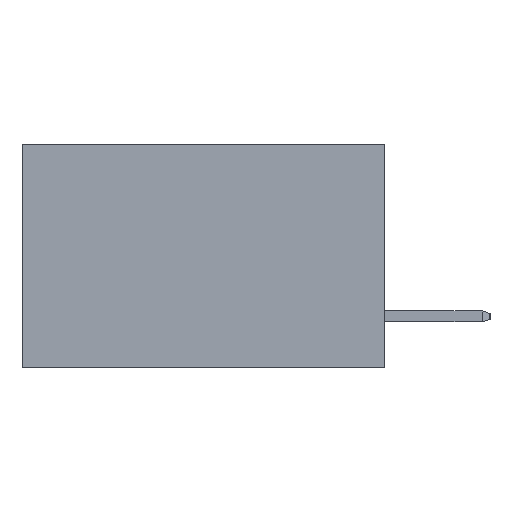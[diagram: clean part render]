
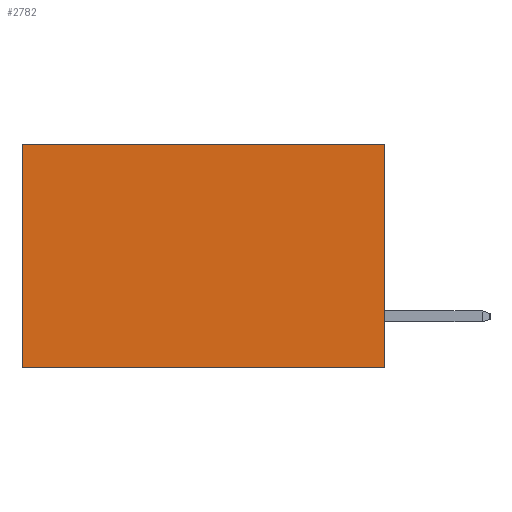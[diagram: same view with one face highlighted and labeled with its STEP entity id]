
A CAD part, left-side view. The second image highlights one B-rep face of the part: STEP entity #2782.
In plain terms, the highlighted planar face has unit normal (-1, 0, 0).
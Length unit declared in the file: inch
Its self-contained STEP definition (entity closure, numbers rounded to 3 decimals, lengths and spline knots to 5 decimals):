
#488 = VECTOR ( 'NONE', #8512, 39.37008 ) ;
#619 = VECTOR ( 'NONE', #1929, 39.37008 ) ;
#1656 = EDGE_CURVE ( 'NONE', #5287, #8365, #6514, .T. ) ;
#1929 = DIRECTION ( 'NONE',  ( 0., 0., -1. ) ) ;
#2061 = DIRECTION ( 'NONE',  ( 0., 1., 0. ) ) ;
#2782 = ADVANCED_FACE ( 'NONE', ( #6607 ), #8817, .F. ) ;
#2809 = EDGE_CURVE ( 'NONE', #6553, #5287, #4385, .T. ) ;
#2838 = CARTESIAN_POINT ( 'NONE',  ( 0.2615, 0.6, -0.37 ) ) ;
#3063 = ORIENTED_EDGE ( 'NONE', *, *, #1656, .T. ) ;
#3164 = ORIENTED_EDGE ( 'NONE', *, *, #7146, .F. ) ;
#3198 = ORIENTED_EDGE ( 'NONE', *, *, #4214, .F. ) ;
#3454 = ORIENTED_EDGE ( 'NONE', *, *, #2809, .T. ) ;
#4123 = LINE ( 'NONE', #7070, #8894 ) ;
#4208 = VERTEX_POINT ( 'NONE', #4673 ) ;
#4214 = EDGE_CURVE ( 'NONE', #6553, #4208, #6358, .T. ) ;
#4385 = LINE ( 'NONE', #8530, #488 ) ;
#4673 = CARTESIAN_POINT ( 'NONE',  ( 0.2615, 0., -0.37 ) ) ;
#5009 = CARTESIAN_POINT ( 'NONE',  ( 0.2615, 0.6, 0. ) ) ;
#5287 = VERTEX_POINT ( 'NONE', #5009 ) ;
#5391 = CARTESIAN_POINT ( 'NONE',  ( 0.2615, 0., -0.37 ) ) ;
#6055 = DIRECTION ( 'NONE',  ( 0., 0., -1. ) ) ;
#6171 = VECTOR ( 'NONE', #6055, 39.37008 ) ;
#6358 = LINE ( 'NONE', #5391, #6171 ) ;
#6514 = LINE ( 'NONE', #7064, #619 ) ;
#6553 = VERTEX_POINT ( 'NONE', #8529 ) ;
#6607 = FACE_OUTER_BOUND ( 'NONE', #6918, .T. ) ;
#6918 = EDGE_LOOP ( 'NONE', ( #3063, #3164, #3198, #3454 ) ) ;
#7064 = CARTESIAN_POINT ( 'NONE',  ( 0.2615, 0.6, -0.37 ) ) ;
#7070 = CARTESIAN_POINT ( 'NONE',  ( 0.2615, 0., -0.37 ) ) ;
#7146 = EDGE_CURVE ( 'NONE', #4208, #8365, #4123, .T. ) ;
#7281 = AXIS2_PLACEMENT_3D ( 'NONE', #8864, #8801, #8782 ) ;
#8365 = VERTEX_POINT ( 'NONE', #2838 ) ;
#8512 = DIRECTION ( 'NONE',  ( 0., 1., 0. ) ) ;
#8529 = CARTESIAN_POINT ( 'NONE',  ( 0.2615, 0., 0. ) ) ;
#8530 = CARTESIAN_POINT ( 'NONE',  ( 0.2615, 0., 0. ) ) ;
#8782 = DIRECTION ( 'NONE',  ( 0., 0., -1. ) ) ;
#8801 = DIRECTION ( 'NONE',  ( 1., 0., 0. ) ) ;
#8817 = PLANE ( 'NONE',  #7281 ) ;
#8864 = CARTESIAN_POINT ( 'NONE',  ( 0.2615, 0., -0.37 ) ) ;
#8894 = VECTOR ( 'NONE', #2061, 39.37008 ) ;
